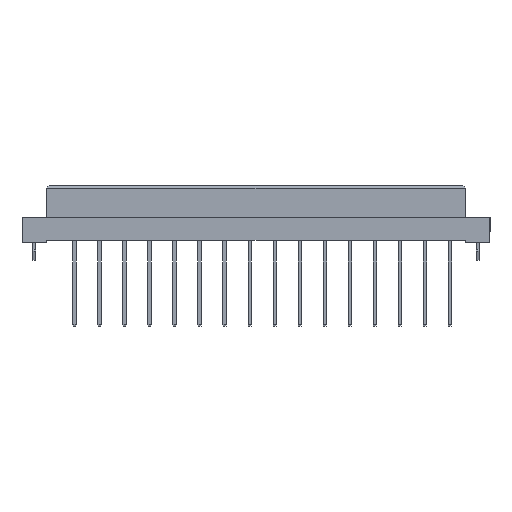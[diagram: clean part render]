
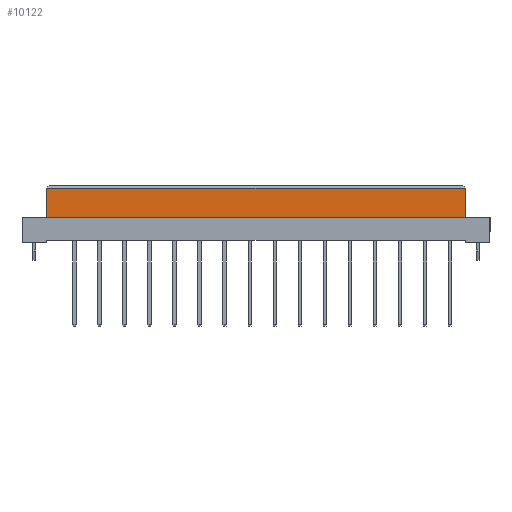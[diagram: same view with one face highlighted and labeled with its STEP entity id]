
A CAD part, top view. The second image highlights one B-rep face of the part: STEP entity #10122.
In plain terms, the highlighted planar face has unit normal (0, 0, 1).
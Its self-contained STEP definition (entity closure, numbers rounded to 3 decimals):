
#1436 = EDGE_LOOP ( 'NONE', ( #9498, #20175, #30648, #38136 ) ) ;
#2800 = AXIS2_PLACEMENT_3D ( 'NONE', #16211, #25642, #22704 ) ;
#3721 = DIRECTION ( 'NONE',  ( -1., 0., 0. ) ) ;
#4539 = CARTESIAN_POINT ( 'NONE',  ( -42.5, -0.5, 4.25 ) ) ;
#5458 = VECTOR ( 'NONE', #18178, 1000. ) ;
#7274 = EDGE_CURVE ( 'NONE', #30831, #21086, #17782, .T. ) ;
#9498 = ORIENTED_EDGE ( 'NONE', *, *, #29522, .T. ) ;
#10122 = ADVANCED_FACE ( 'NONE', ( #10700 ), #31728, .T. ) ;
#10700 = FACE_OUTER_BOUND ( 'NONE', #1436, .T. ) ;
#10923 = VERTEX_POINT ( 'NONE', #34323 ) ;
#11588 = EDGE_CURVE ( 'NONE', #30831, #10923, #31537, .T. ) ;
#12241 = LINE ( 'NONE', #24450, #5458 ) ;
#12951 = VECTOR ( 'NONE', #31727, 1000. ) ;
#16211 = CARTESIAN_POINT ( 'NONE',  ( 42.5, -6.4, 4.25 ) ) ;
#17782 = LINE ( 'NONE', #26623, #24358 ) ;
#17784 = EDGE_CURVE ( 'NONE', #25540, #21086, #24965, .T. ) ;
#18178 = DIRECTION ( 'NONE',  ( 0., 1., 0. ) ) ;
#19955 = CARTESIAN_POINT ( 'NONE',  ( -42.5, -6.4, 4.25 ) ) ;
#20175 = ORIENTED_EDGE ( 'NONE', *, *, #17784, .T. ) ;
#21086 = VERTEX_POINT ( 'NONE', #4539 ) ;
#22704 = DIRECTION ( 'NONE',  ( 1., 0., 0. ) ) ;
#23281 = CARTESIAN_POINT ( 'NONE',  ( 42.5, -6.4, 4.25 ) ) ;
#24358 = VECTOR ( 'NONE', #26822, 1000. ) ;
#24450 = CARTESIAN_POINT ( 'NONE',  ( 42.5, -6.4, 4.25 ) ) ;
#24965 = LINE ( 'NONE', #30669, #37025 ) ;
#25540 = VERTEX_POINT ( 'NONE', #34126 ) ;
#25642 = DIRECTION ( 'NONE',  ( 0., 0., 1. ) ) ;
#26623 = CARTESIAN_POINT ( 'NONE',  ( -42.5, -6.4, 4.25 ) ) ;
#26822 = DIRECTION ( 'NONE',  ( 0., 1., 0. ) ) ;
#29522 = EDGE_CURVE ( 'NONE', #10923, #25540, #12241, .T. ) ;
#30648 = ORIENTED_EDGE ( 'NONE', *, *, #7274, .F. ) ;
#30669 = CARTESIAN_POINT ( 'NONE',  ( -42.5, -0.5, 4.25 ) ) ;
#30831 = VERTEX_POINT ( 'NONE', #19955 ) ;
#31537 = LINE ( 'NONE', #23281, #12951 ) ;
#31727 = DIRECTION ( 'NONE',  ( 1., 0., 0. ) ) ;
#31728 = PLANE ( 'NONE',  #2800 ) ;
#34126 = CARTESIAN_POINT ( 'NONE',  ( 42.5, -0.5, 4.25 ) ) ;
#34323 = CARTESIAN_POINT ( 'NONE',  ( 42.5, -6.4, 4.25 ) ) ;
#37025 = VECTOR ( 'NONE', #3721, 1000. ) ;
#38136 = ORIENTED_EDGE ( 'NONE', *, *, #11588, .T. ) ;
